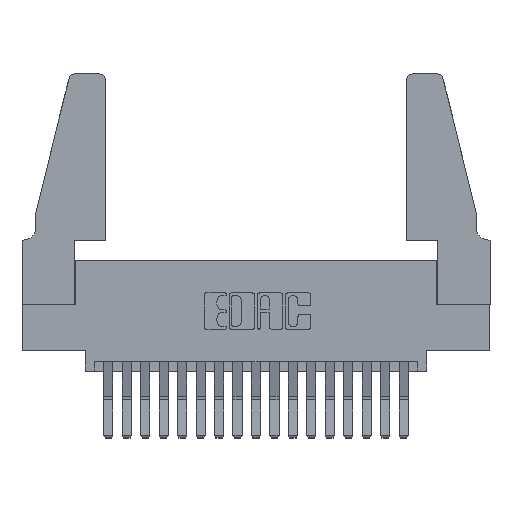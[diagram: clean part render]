
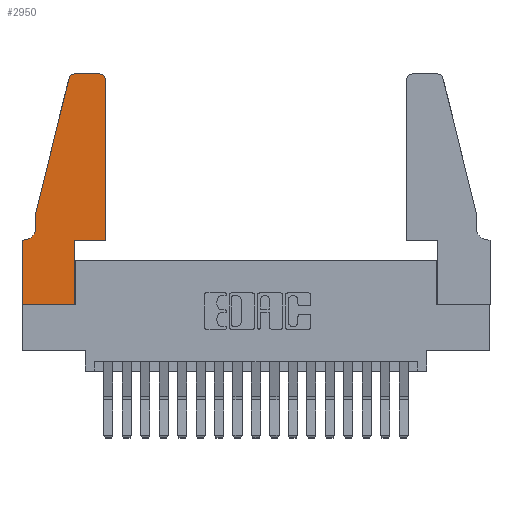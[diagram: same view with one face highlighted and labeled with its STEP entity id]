
A CAD part, top view. The second image highlights one B-rep face of the part: STEP entity #2950.
In plain terms, the highlighted planar face has unit normal (0, 0, 1).
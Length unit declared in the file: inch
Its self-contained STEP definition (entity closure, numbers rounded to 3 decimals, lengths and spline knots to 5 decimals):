
#121 = ORIENTED_EDGE ( 'NONE', *, *, #13414, .T. ) ;
#477 = VECTOR ( 'NONE', #1913, 39.37008 ) ;
#950 = EDGE_CURVE ( 'NONE', #12489, #8377, #6898, .T. ) ;
#1602 = CARTESIAN_POINT ( 'NONE',  ( 0.0755, 0.5, 0.37 ) ) ;
#1820 = AXIS2_PLACEMENT_3D ( 'NONE', #2739, #13102, #4289 ) ;
#1878 = LINE ( 'NONE', #6767, #17951 ) ;
#1885 = DIRECTION ( 'NONE',  ( 0., 0., -1. ) ) ;
#1910 = VERTEX_POINT ( 'NONE', #15336 ) ;
#1913 = DIRECTION ( 'NONE',  ( 1., 0., 0. ) ) ;
#1995 = VECTOR ( 'NONE', #3686, 39.37008 ) ;
#2165 = DIRECTION ( 'NONE',  ( 0., 0., 1. ) ) ;
#2512 = VECTOR ( 'NONE', #17438, 39.37008 ) ;
#2565 = ORIENTED_EDGE ( 'NONE', *, *, #15190, .T. ) ;
#2585 = ORIENTED_EDGE ( 'NONE', *, *, #13363, .T. ) ;
#2705 = CARTESIAN_POINT ( 'NONE',  ( 0.4505, 0.35, 0.37 ) ) ;
#2739 = CARTESIAN_POINT ( 'NONE',  ( 0.284, 1.22, 0.37 ) ) ;
#2853 = LINE ( 'NONE', #11796, #11227 ) ;
#2939 = AXIS2_PLACEMENT_3D ( 'NONE', #11089, #2165, #12534 ) ;
#2950 = ADVANCED_FACE ( 'NONE', ( #7790 ), #17519, .T. ) ;
#3175 = EDGE_CURVE ( 'NONE', #12231, #12489, #5480, .T. ) ;
#3686 = DIRECTION ( 'NONE',  ( -1., 0., 0. ) ) ;
#3805 = VECTOR ( 'NONE', #4320, 39.37008 ) ;
#3945 = ORIENTED_EDGE ( 'NONE', *, *, #7614, .T. ) ;
#4044 = EDGE_CURVE ( 'NONE', #12988, #5305, #1878, .T. ) ;
#4289 = DIRECTION ( 'NONE',  ( 1., 0., 0. ) ) ;
#4320 = DIRECTION ( 'NONE',  ( 0., -1., 0. ) ) ;
#4417 = ORIENTED_EDGE ( 'NONE', *, *, #950, .T. ) ;
#4448 = DIRECTION ( 'NONE',  ( 0., 1., 0. ) ) ;
#4697 = EDGE_LOOP ( 'NONE', ( #3945, #11956, #17077, #18103, #2565, #12654, #2585, #6691, #4417, #9431, #121, #12311 ) ) ;
#5085 = VERTEX_POINT ( 'NONE', #17053 ) ;
#5115 = LINE ( 'NONE', #15004, #12474 ) ;
#5305 = VERTEX_POINT ( 'NONE', #11791 ) ;
#5480 = LINE ( 'NONE', #18015, #477 ) ;
#5587 = AXIS2_PLACEMENT_3D ( 'NONE', #10829, #1885, #12281 ) ;
#6046 = LINE ( 'NONE', #11090, #1995 ) ;
#6092 = LINE ( 'NONE', #8801, #2512 ) ;
#6158 = VECTOR ( 'NONE', #17362, 39.37008 ) ;
#6455 = CARTESIAN_POINT ( 'NONE',  ( 0.4205, 1.25, 0.37 ) ) ;
#6691 = ORIENTED_EDGE ( 'NONE', *, *, #3175, .T. ) ;
#6767 = CARTESIAN_POINT ( 'NONE',  ( 0.0755, 0.5, 0.37 ) ) ;
#6777 = EDGE_CURVE ( 'NONE', #5085, #12988, #5115, .T. ) ;
#6837 = CIRCLE ( 'NONE', #2939, 0.03 ) ;
#6898 = LINE ( 'NONE', #9883, #14188 ) ;
#6969 = CARTESIAN_POINT ( 'NONE',  ( 0.284, 1.25, 0.37 ) ) ;
#7146 = VERTEX_POINT ( 'NONE', #2705 ) ;
#7614 = EDGE_CURVE ( 'NONE', #8177, #14784, #6046, .T. ) ;
#7776 = LINE ( 'NONE', #14568, #3805 ) ;
#7790 = FACE_OUTER_BOUND ( 'NONE', #4697, .T. ) ;
#7868 = EDGE_CURVE ( 'NONE', #13349, #1910, #17715, .T. ) ;
#8177 = VERTEX_POINT ( 'NONE', #6455 ) ;
#8377 = VERTEX_POINT ( 'NONE', #14146 ) ;
#8801 = CARTESIAN_POINT ( 'NONE',  ( 0.4505, 0.35, 0.37 ) ) ;
#8959 = CARTESIAN_POINT ( 'NONE',  ( 0., 0.35, 0.37 ) ) ;
#9214 = EDGE_CURVE ( 'NONE', #8377, #7146, #6092, .T. ) ;
#9431 = ORIENTED_EDGE ( 'NONE', *, *, #9214, .T. ) ;
#9882 = EDGE_CURVE ( 'NONE', #14784, #5085, #17859, .T. ) ;
#9883 = CARTESIAN_POINT ( 'NONE',  ( 0.2865, 0.35, 0.37 ) ) ;
#10416 = DIRECTION ( 'NONE',  ( 1., 0., 0. ) ) ;
#10702 = AXIS2_PLACEMENT_3D ( 'NONE', #8959, #19060, #10416 ) ;
#10829 = CARTESIAN_POINT ( 'NONE',  ( 0.0055, 0.42, 0.37 ) ) ;
#11089 = CARTESIAN_POINT ( 'NONE',  ( 0.4205, 1.22, 0.37 ) ) ;
#11090 = CARTESIAN_POINT ( 'NONE',  ( 0.2605, 1.25, 0.37 ) ) ;
#11227 = VECTOR ( 'NONE', #4448, 39.37008 ) ;
#11366 = DIRECTION ( 'NONE',  ( 0., 1., 0. ) ) ;
#11617 = VERTEX_POINT ( 'NONE', #11929 ) ;
#11679 = CARTESIAN_POINT ( 'NONE',  ( 0.0055, 0.35, 0.37 ) ) ;
#11791 = CARTESIAN_POINT ( 'NONE',  ( 0.0755, 0.42, 0.37 ) ) ;
#11796 = CARTESIAN_POINT ( 'NONE',  ( 0.4505, 0.35, 0.37 ) ) ;
#11929 = CARTESIAN_POINT ( 'NONE',  ( 0.4505, 1.22, 0.37 ) ) ;
#11956 = ORIENTED_EDGE ( 'NONE', *, *, #9882, .T. ) ;
#12231 = VERTEX_POINT ( 'NONE', #13230 ) ;
#12281 = DIRECTION ( 'NONE',  ( -1., 0., 0. ) ) ;
#12311 = ORIENTED_EDGE ( 'NONE', *, *, #16659, .T. ) ;
#12474 = VECTOR ( 'NONE', #17904, 39.37008 ) ;
#12489 = VERTEX_POINT ( 'NONE', #16589 ) ;
#12534 = DIRECTION ( 'NONE',  ( 1., 0., 0. ) ) ;
#12654 = ORIENTED_EDGE ( 'NONE', *, *, #7868, .T. ) ;
#12988 = VERTEX_POINT ( 'NONE', #1602 ) ;
#13102 = DIRECTION ( 'NONE',  ( 0., 0., 1. ) ) ;
#13230 = CARTESIAN_POINT ( 'NONE',  ( 0., 0., 0.37 ) ) ;
#13349 = VERTEX_POINT ( 'NONE', #11679 ) ;
#13363 = EDGE_CURVE ( 'NONE', #1910, #12231, #7776, .T. ) ;
#13414 = EDGE_CURVE ( 'NONE', #7146, #11617, #2853, .T. ) ;
#14146 = CARTESIAN_POINT ( 'NONE',  ( 0.2865, 0.35, 0.37 ) ) ;
#14188 = VECTOR ( 'NONE', #11366, 39.37008 ) ;
#14484 = CARTESIAN_POINT ( 'NONE',  ( 0.0755, 0.35, 0.37 ) ) ;
#14568 = CARTESIAN_POINT ( 'NONE',  ( 0., 0., 0.37 ) ) ;
#14784 = VERTEX_POINT ( 'NONE', #6969 ) ;
#15004 = CARTESIAN_POINT ( 'NONE',  ( 0.0755, 0.5, 0.37 ) ) ;
#15190 = EDGE_CURVE ( 'NONE', #5305, #13349, #15969, .T. ) ;
#15336 = CARTESIAN_POINT ( 'NONE',  ( 0., 0.35, 0.37 ) ) ;
#15969 = CIRCLE ( 'NONE', #5587, 0.07 ) ;
#16589 = CARTESIAN_POINT ( 'NONE',  ( 0.2865, 0., 0.37 ) ) ;
#16659 = EDGE_CURVE ( 'NONE', #11617, #8177, #6837, .T. ) ;
#17053 = CARTESIAN_POINT ( 'NONE',  ( 0.25487, 1.22718, 0.37 ) ) ;
#17077 = ORIENTED_EDGE ( 'NONE', *, *, #6777, .T. ) ;
#17362 = DIRECTION ( 'NONE',  ( -1., 0., 0. ) ) ;
#17438 = DIRECTION ( 'NONE',  ( 1., 0., 0. ) ) ;
#17519 = PLANE ( 'NONE',  #10702 ) ;
#17715 = LINE ( 'NONE', #14484, #6158 ) ;
#17859 = CIRCLE ( 'NONE', #1820, 0.03 ) ;
#17904 = DIRECTION ( 'NONE',  ( -0.239, -0.971, 0. ) ) ;
#17951 = VECTOR ( 'NONE', #18316, 39.37008 ) ;
#18015 = CARTESIAN_POINT ( 'NONE',  ( 0., 0., 0.37 ) ) ;
#18103 = ORIENTED_EDGE ( 'NONE', *, *, #4044, .T. ) ;
#18316 = DIRECTION ( 'NONE',  ( 0., -1., 0. ) ) ;
#19060 = DIRECTION ( 'NONE',  ( 0., 0., 1. ) ) ;
